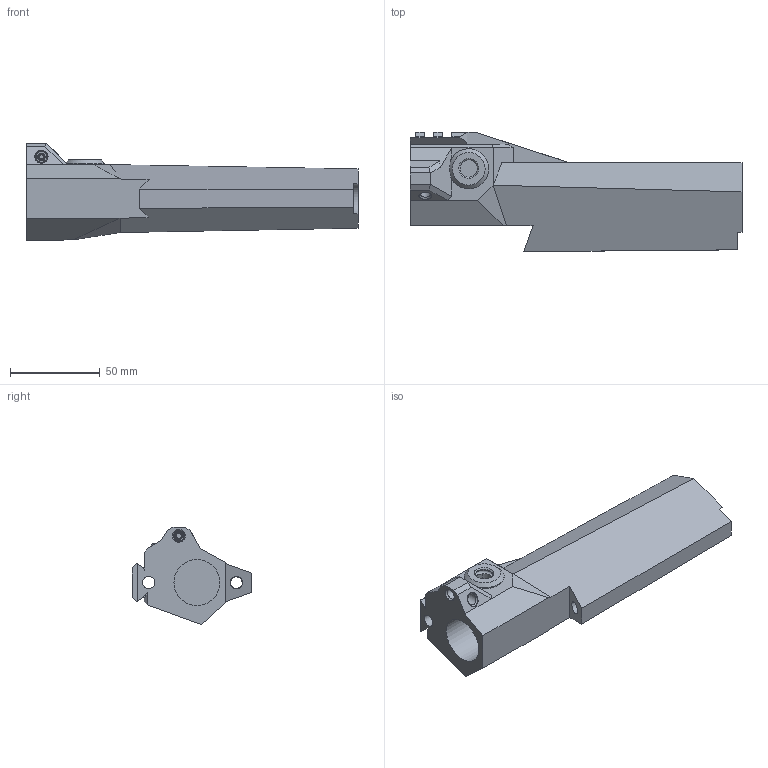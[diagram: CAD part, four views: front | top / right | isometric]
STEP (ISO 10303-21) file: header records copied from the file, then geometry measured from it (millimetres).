
FILE_DESCRIPTION(/* description */ (''),/* implementation_level */ '2;1');
FILE_NAME(/* name */ 'ARK Chargin'' Handle/BUFFER TUBE.step',/* time_stamp */ '2022-02-02T21:14:59-07:00',/* author */ (''),/* organization */ (''),/* preprocessor_version */ 'ST-DEVELOPER v18.1',/* originating_system */ 'Autodesk Translation Framework v10.13.0.1454',/* authorisation */ '');
FILE_SCHEMA (('AUTOMOTIVE_DESIGN { 1 0 10303 214 3 1 1 }'));
Length unit declared in the file: millimetre
Products named in the file (1): BUFFER TUBE
Bounding box: 184.46 x 66.32 x 54.14 mm (x, y, z)
Volume: 149006.7 mm3; surface area: 50391.1 mm2
Topology: 1 solids, 2 shells, 157 faces, 415 edges, 270 vertices
Faces by surface type: plane 112, bspline 18, cylinder 13, torus 9, cone 5
Full cylindrical faces by diameter (mm): 2.8 x1, 3 x1, 6 x2, 6.85 x1, 9.2 x1, 9.6 x1, 25.546 x1
Entity records: 5587 total; most frequent: CARTESIAN_POINT 1719, ORIENTED_EDGE 830, DIRECTION 719, EDGE_CURVE 415, LINE 311, VECTOR 311, VERTEX_POINT 270, AXIS2_PLACEMENT_3D 204
